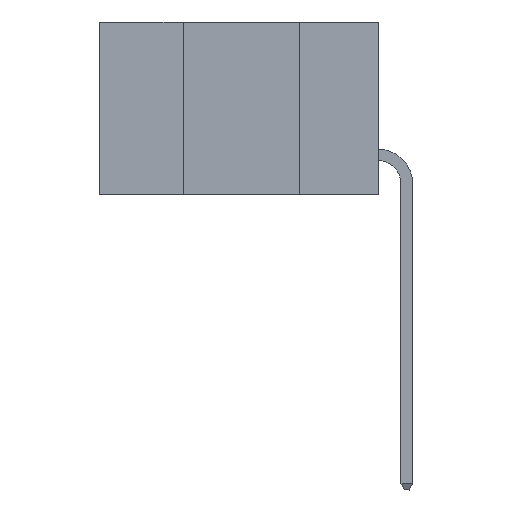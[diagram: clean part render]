
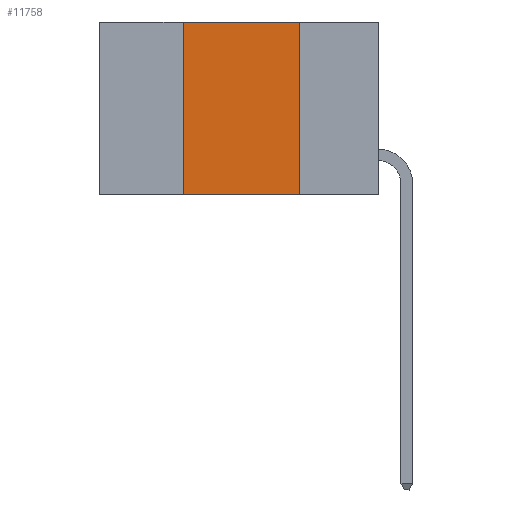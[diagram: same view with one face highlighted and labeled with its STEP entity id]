
A CAD part, left-side view. The second image highlights one B-rep face of the part: STEP entity #11758.
In plain terms, the highlighted planar face has unit normal (-1, 0, 0).
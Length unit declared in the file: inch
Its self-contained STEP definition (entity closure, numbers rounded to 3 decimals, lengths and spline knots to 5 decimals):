
#933 = LINE ( 'NONE', #3927, #9700 ) ;
#1010 = CARTESIAN_POINT ( 'NONE',  ( 0., 0.6, 0. ) ) ;
#1101 = AXIS2_PLACEMENT_3D ( 'NONE', #11640, #12445, #8586 ) ;
#1471 = EDGE_LOOP ( 'NONE', ( #3620, #9369, #6535, #12985 ) ) ;
#1748 = DIRECTION ( 'NONE',  ( 0., -1., 0. ) ) ;
#2230 = PLANE ( 'NONE',  #1101 ) ;
#2563 = CARTESIAN_POINT ( 'NONE',  ( 0., 0.17, -0.37 ) ) ;
#2597 = LINE ( 'NONE', #4631, #3681 ) ;
#3252 = LINE ( 'NONE', #10339, #6482 ) ;
#3620 = ORIENTED_EDGE ( 'NONE', *, *, #10531, .F. ) ;
#3681 = VECTOR ( 'NONE', #13072, 39.37008 ) ;
#3707 = VERTEX_POINT ( 'NONE', #5299 ) ;
#3725 = VERTEX_POINT ( 'NONE', #5373 ) ;
#3927 = CARTESIAN_POINT ( 'NONE',  ( 0., 0.6, -0.37 ) ) ;
#4631 = CARTESIAN_POINT ( 'NONE',  ( 0., 0.42, -0.37 ) ) ;
#4720 = VERTEX_POINT ( 'NONE', #9414 ) ;
#5299 = CARTESIAN_POINT ( 'NONE',  ( 0., 0.17, 0. ) ) ;
#5373 = CARTESIAN_POINT ( 'NONE',  ( 0., 0.42, 0. ) ) ;
#5484 = FACE_OUTER_BOUND ( 'NONE', #1471, .T. ) ;
#6091 = LINE ( 'NONE', #1010, #10594 ) ;
#6482 = VECTOR ( 'NONE', #10473, 39.37008 ) ;
#6535 = ORIENTED_EDGE ( 'NONE', *, *, #10104, .F. ) ;
#6911 = DIRECTION ( 'NONE',  ( 0., -1., 0. ) ) ;
#8586 = DIRECTION ( 'NONE',  ( 0., 0., -1. ) ) ;
#9276 = EDGE_CURVE ( 'NONE', #4720, #12410, #933, .T. ) ;
#9369 = ORIENTED_EDGE ( 'NONE', *, *, #10435, .F. ) ;
#9414 = CARTESIAN_POINT ( 'NONE',  ( 0., 0.42, -0.37 ) ) ;
#9700 = VECTOR ( 'NONE', #1748, 39.37008 ) ;
#10104 = EDGE_CURVE ( 'NONE', #4720, #3725, #2597, .T. ) ;
#10339 = CARTESIAN_POINT ( 'NONE',  ( 0., 0.17, -0.37 ) ) ;
#10435 = EDGE_CURVE ( 'NONE', #3725, #3707, #6091, .T. ) ;
#10473 = DIRECTION ( 'NONE',  ( 0., 0., -1. ) ) ;
#10531 = EDGE_CURVE ( 'NONE', #3707, #12410, #3252, .T. ) ;
#10594 = VECTOR ( 'NONE', #6911, 39.37008 ) ;
#11640 = CARTESIAN_POINT ( 'NONE',  ( 0., 0.6, 0. ) ) ;
#11758 = ADVANCED_FACE ( 'NONE', ( #5484 ), #2230, .F. ) ;
#12410 = VERTEX_POINT ( 'NONE', #2563 ) ;
#12445 = DIRECTION ( 'NONE',  ( 1., 0., 0. ) ) ;
#12985 = ORIENTED_EDGE ( 'NONE', *, *, #9276, .T. ) ;
#13072 = DIRECTION ( 'NONE',  ( 0., 0., 1. ) ) ;
